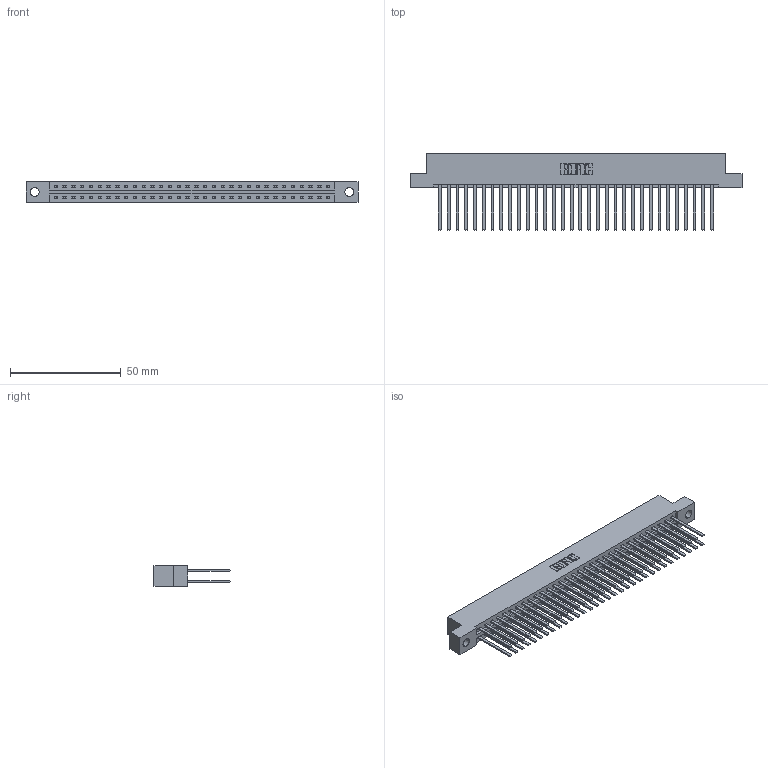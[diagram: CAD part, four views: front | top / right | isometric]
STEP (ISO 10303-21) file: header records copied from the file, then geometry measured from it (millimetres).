
FILE_DESCRIPTION (( 'STEP AP203' ), '1' );
FILE_NAME ('387-064-544-204.STEP', '2019-10-19T17:03:02', ( '' ), ( '' ), 'SwSTEP 2.0', 'SolidWorks 2016', '' );
FILE_SCHEMA (( 'CONFIG_CONTROL_DESIGN' ));
Length unit declared in the file: inch
Products named in the file (3): 345-292-001_345-293-144; 337 Part_Flush Mounting Lugs - 0.156 Dia-TH; 387-064-544-204
Assembly tree (65 placements, depth 2):
  387-064-544-204
    337 Part_Flush Mounting Lugs - 0.156 Dia-TH
    345-292-001_345-293-144  x64
Bounding box: 149.81 x 34.3 x 9.4 mm (x, y, z)
Volume: 16464.3 mm3; surface area: 21243.9 mm2
Topology: 65 solids, 65 shells, 3186 faces, 9463 edges, 6222 vertices
Faces by surface type: plane 2246, cylinder 940
Entity records: 25923 total; most frequent: CARTESIAN_POINT 4374, ORIENTED_EDGE 4310, DIRECTION 3735, EDGE_CURVE 2155, LINE 2031, VECTOR 2031, VERTEX_POINT 1434, AXIS2_PLACEMENT_3D 852
